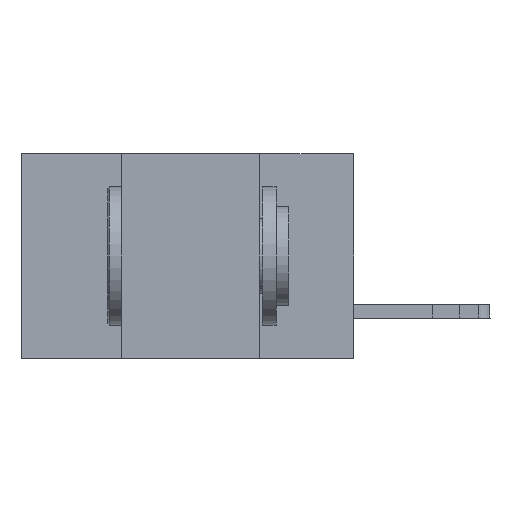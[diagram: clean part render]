
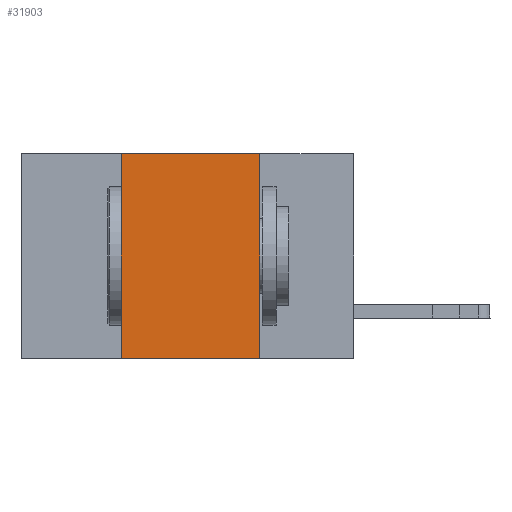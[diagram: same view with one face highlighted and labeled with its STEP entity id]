
A CAD part, left-side view. The second image highlights one B-rep face of the part: STEP entity #31903.
In plain terms, the highlighted planar face has unit normal (-1, 0, 0).
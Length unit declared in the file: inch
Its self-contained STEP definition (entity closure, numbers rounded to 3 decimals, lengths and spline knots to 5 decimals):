
#185 = LINE ( 'NONE', #18739, #2108 ) ;
#613 = LINE ( 'NONE', #15796, #3960 ) ;
#2108 = VECTOR ( 'NONE', #3241, 39.37008 ) ;
#3241 = DIRECTION ( 'NONE',  ( 0., 0., -1. ) ) ;
#3960 = VECTOR ( 'NONE', #31227, 39.37008 ) ;
#4958 = AXIS2_PLACEMENT_3D ( 'NONE', #5388, #8465, #29924 ) ;
#5388 = CARTESIAN_POINT ( 'NONE',  ( 0., 0.6, 0. ) ) ;
#5633 = CARTESIAN_POINT ( 'NONE',  ( 0., 0.6, 0. ) ) ;
#6907 = CARTESIAN_POINT ( 'NONE',  ( 0., 0.42, 0. ) ) ;
#7556 = ORIENTED_EDGE ( 'NONE', *, *, #14010, .F. ) ;
#8465 = DIRECTION ( 'NONE',  ( 1., 0., 0. ) ) ;
#9279 = EDGE_CURVE ( 'NONE', #14260, #29610, #613, .T. ) ;
#11214 = FACE_OUTER_BOUND ( 'NONE', #31068, .T. ) ;
#11783 = EDGE_CURVE ( 'NONE', #18583, #27490, #35833, .T. ) ;
#11786 = DIRECTION ( 'NONE',  ( 0., -1., 0. ) ) ;
#14010 = EDGE_CURVE ( 'NONE', #14260, #18583, #21686, .T. ) ;
#14260 = VERTEX_POINT ( 'NONE', #29104 ) ;
#15796 = CARTESIAN_POINT ( 'NONE',  ( 0., 0.6, -0.37 ) ) ;
#18583 = VERTEX_POINT ( 'NONE', #19396 ) ;
#18739 = CARTESIAN_POINT ( 'NONE',  ( 0., 0.17, 0. ) ) ;
#18904 = ORIENTED_EDGE ( 'NONE', *, *, #9279, .T. ) ;
#19222 = CARTESIAN_POINT ( 'NONE',  ( 0., 0.17, 0. ) ) ;
#19396 = CARTESIAN_POINT ( 'NONE',  ( 0., 0.42, 0. ) ) ;
#21348 = ORIENTED_EDGE ( 'NONE', *, *, #31916, .F. ) ;
#21686 = LINE ( 'NONE', #6907, #26938 ) ;
#23462 = ORIENTED_EDGE ( 'NONE', *, *, #11783, .F. ) ;
#26938 = VECTOR ( 'NONE', #28734, 39.37008 ) ;
#27490 = VERTEX_POINT ( 'NONE', #19222 ) ;
#28734 = DIRECTION ( 'NONE',  ( 0., 0., 1. ) ) ;
#29104 = CARTESIAN_POINT ( 'NONE',  ( 0., 0.42, -0.37 ) ) ;
#29285 = CARTESIAN_POINT ( 'NONE',  ( 0., 0.17, -0.37 ) ) ;
#29610 = VERTEX_POINT ( 'NONE', #29285 ) ;
#29924 = DIRECTION ( 'NONE',  ( 0., 0., -1. ) ) ;
#31068 = EDGE_LOOP ( 'NONE', ( #21348, #23462, #7556, #18904 ) ) ;
#31227 = DIRECTION ( 'NONE',  ( 0., -1., 0. ) ) ;
#31903 = ADVANCED_FACE ( 'NONE', ( #11214 ), #39463, .F. ) ;
#31916 = EDGE_CURVE ( 'NONE', #27490, #29610, #185, .T. ) ;
#34863 = VECTOR ( 'NONE', #11786, 39.37008 ) ;
#35833 = LINE ( 'NONE', #5633, #34863 ) ;
#39463 = PLANE ( 'NONE',  #4958 ) ;
